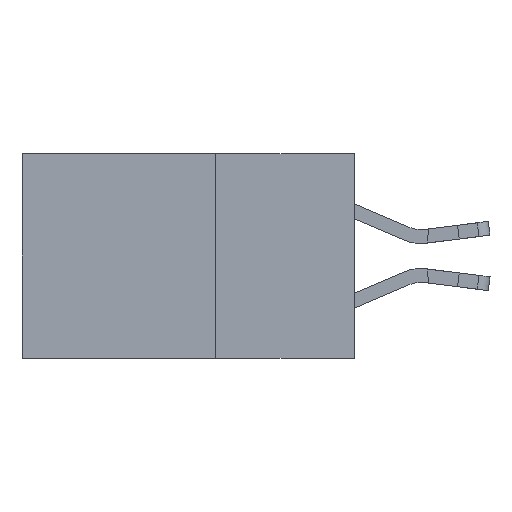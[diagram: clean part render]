
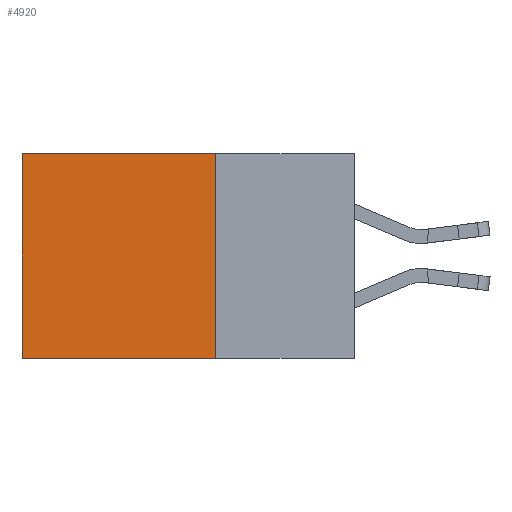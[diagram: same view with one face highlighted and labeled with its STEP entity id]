
A CAD part, left-side view. The second image highlights one B-rep face of the part: STEP entity #4920.
In plain terms, the highlighted planar face has unit normal (-1, 0, 0).
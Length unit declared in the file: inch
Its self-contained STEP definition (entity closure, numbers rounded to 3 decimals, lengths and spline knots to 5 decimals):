
#320 = EDGE_CURVE ( 'NONE', #11646, #15211, #13015, .T. ) ;
#606 = EDGE_CURVE ( 'NONE', #8116, #15211, #5071, .T. ) ;
#1014 = LINE ( 'NONE', #15140, #13243 ) ;
#1125 = DIRECTION ( 'NONE',  ( 0., 0., -1. ) ) ;
#2254 = DIRECTION ( 'NONE',  ( 0., 0., -1. ) ) ;
#2439 = CARTESIAN_POINT ( 'NONE',  ( 0.298, 0.25, 0. ) ) ;
#3374 = ORIENTED_EDGE ( 'NONE', *, *, #606, .F. ) ;
#3604 = VERTEX_POINT ( 'NONE', #12851 ) ;
#3737 = DIRECTION ( 'NONE',  ( 0., 1., 0. ) ) ;
#4920 = ADVANCED_FACE ( 'NONE', ( #13379 ), #14489, .F. ) ;
#4997 = DIRECTION ( 'NONE',  ( 1., 0., 0. ) ) ;
#5071 = LINE ( 'NONE', #11811, #14122 ) ;
#5736 = VECTOR ( 'NONE', #1125, 39.37008 ) ;
#6225 = CARTESIAN_POINT ( 'NONE',  ( 0.298, 0.25, 0. ) ) ;
#6932 = AXIS2_PLACEMENT_3D ( 'NONE', #6225, #4997, #11986 ) ;
#7613 = LINE ( 'NONE', #2439, #5736 ) ;
#8116 = VERTEX_POINT ( 'NONE', #15349 ) ;
#8447 = ORIENTED_EDGE ( 'NONE', *, *, #14057, .T. ) ;
#8880 = ORIENTED_EDGE ( 'NONE', *, *, #320, .T. ) ;
#9162 = DIRECTION ( 'NONE',  ( 0., 1., 0. ) ) ;
#10376 = ORIENTED_EDGE ( 'NONE', *, *, #11894, .F. ) ;
#11243 = EDGE_LOOP ( 'NONE', ( #8880, #3374, #10376, #8447 ) ) ;
#11646 = VERTEX_POINT ( 'NONE', #12292 ) ;
#11736 = VECTOR ( 'NONE', #2254, 39.37008 ) ;
#11811 = CARTESIAN_POINT ( 'NONE',  ( 0.298, 0.25, -0.37 ) ) ;
#11887 = CARTESIAN_POINT ( 'NONE',  ( 0.298, 0.6, 0. ) ) ;
#11894 = EDGE_CURVE ( 'NONE', #3604, #8116, #7613, .T. ) ;
#11986 = DIRECTION ( 'NONE',  ( 0., 0., -1. ) ) ;
#12292 = CARTESIAN_POINT ( 'NONE',  ( 0.298, 0.6, 0. ) ) ;
#12851 = CARTESIAN_POINT ( 'NONE',  ( 0.298, 0.25, 0. ) ) ;
#13015 = LINE ( 'NONE', #11887, #11736 ) ;
#13243 = VECTOR ( 'NONE', #9162, 39.37008 ) ;
#13379 = FACE_OUTER_BOUND ( 'NONE', #11243, .T. ) ;
#14057 = EDGE_CURVE ( 'NONE', #3604, #11646, #1014, .T. ) ;
#14122 = VECTOR ( 'NONE', #3737, 39.37008 ) ;
#14482 = CARTESIAN_POINT ( 'NONE',  ( 0.298, 0.6, -0.37 ) ) ;
#14489 = PLANE ( 'NONE',  #6932 ) ;
#15140 = CARTESIAN_POINT ( 'NONE',  ( 0.298, 0.25, 0. ) ) ;
#15211 = VERTEX_POINT ( 'NONE', #14482 ) ;
#15349 = CARTESIAN_POINT ( 'NONE',  ( 0.298, 0.25, -0.37 ) ) ;
